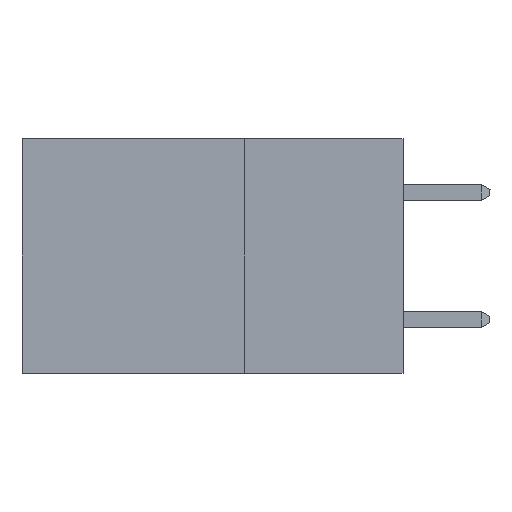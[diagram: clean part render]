
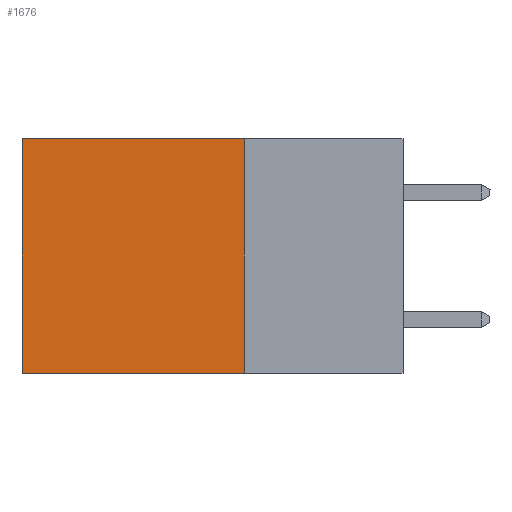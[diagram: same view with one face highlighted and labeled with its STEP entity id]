
A CAD part, left-side view. The second image highlights one B-rep face of the part: STEP entity #1676.
In plain terms, the highlighted planar face has unit normal (-1, 0, 0).
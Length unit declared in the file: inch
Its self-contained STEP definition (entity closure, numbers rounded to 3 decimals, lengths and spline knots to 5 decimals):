
#740 = VERTEX_POINT ( 'NONE', #6843 ) ;
#866 = VECTOR ( 'NONE', #33385, 39.37008 ) ;
#1676 = ADVANCED_FACE ( 'NONE', ( #5299 ), #25380, .F. ) ;
#5062 = DIRECTION ( 'NONE',  ( 0., 0., -1. ) ) ;
#5299 = FACE_OUTER_BOUND ( 'NONE', #20991, .T. ) ;
#5626 = LINE ( 'NONE', #28231, #866 ) ;
#6843 = CARTESIAN_POINT ( 'NONE',  ( 0.2875, 0.25, 0. ) ) ;
#7354 = VECTOR ( 'NONE', #5062, 39.37008 ) ;
#7443 = ORIENTED_EDGE ( 'NONE', *, *, #34254, .F. ) ;
#12840 = ORIENTED_EDGE ( 'NONE', *, *, #30115, .T. ) ;
#12978 = VECTOR ( 'NONE', #23310, 39.37008 ) ;
#13712 = CARTESIAN_POINT ( 'NONE',  ( 0.2875, 0.6, -0.37 ) ) ;
#13892 = CARTESIAN_POINT ( 'NONE',  ( 0.2875, 0.6, 0. ) ) ;
#14160 = CARTESIAN_POINT ( 'NONE',  ( 0.2875, 0.25, 0. ) ) ;
#15309 = DIRECTION ( 'NONE',  ( 0., 0., -1. ) ) ;
#16399 = LINE ( 'NONE', #20783, #12978 ) ;
#19987 = VERTEX_POINT ( 'NONE', #13892 ) ;
#20783 = CARTESIAN_POINT ( 'NONE',  ( 0.2875, 0.25, -0.37 ) ) ;
#20991 = EDGE_LOOP ( 'NONE', ( #12840, #7443, #29085, #34175 ) ) ;
#23310 = DIRECTION ( 'NONE',  ( 0., 1., 0. ) ) ;
#23917 = EDGE_CURVE ( 'NONE', #740, #32586, #31462, .T. ) ;
#24349 = VERTEX_POINT ( 'NONE', #13712 ) ;
#25380 = PLANE ( 'NONE',  #34540 ) ;
#28128 = DIRECTION ( 'NONE',  ( 0., 0., -1. ) ) ;
#28231 = CARTESIAN_POINT ( 'NONE',  ( 0.2875, 0.25, 0. ) ) ;
#29085 = ORIENTED_EDGE ( 'NONE', *, *, #23917, .F. ) ;
#29578 = CARTESIAN_POINT ( 'NONE',  ( 0.2875, 0.6, 0. ) ) ;
#30115 = EDGE_CURVE ( 'NONE', #19987, #24349, #31880, .T. ) ;
#30294 = EDGE_CURVE ( 'NONE', #740, #19987, #5626, .T. ) ;
#30571 = VECTOR ( 'NONE', #15309, 39.37008 ) ;
#31462 = LINE ( 'NONE', #34443, #30571 ) ;
#31880 = LINE ( 'NONE', #29578, #7354 ) ;
#32586 = VERTEX_POINT ( 'NONE', #34143 ) ;
#33385 = DIRECTION ( 'NONE',  ( 0., 1., 0. ) ) ;
#33400 = DIRECTION ( 'NONE',  ( 1., 0., 0. ) ) ;
#34143 = CARTESIAN_POINT ( 'NONE',  ( 0.2875, 0.25, -0.37 ) ) ;
#34175 = ORIENTED_EDGE ( 'NONE', *, *, #30294, .T. ) ;
#34254 = EDGE_CURVE ( 'NONE', #32586, #24349, #16399, .T. ) ;
#34443 = CARTESIAN_POINT ( 'NONE',  ( 0.2875, 0.25, 0. ) ) ;
#34540 = AXIS2_PLACEMENT_3D ( 'NONE', #14160, #33400, #28128 ) ;
